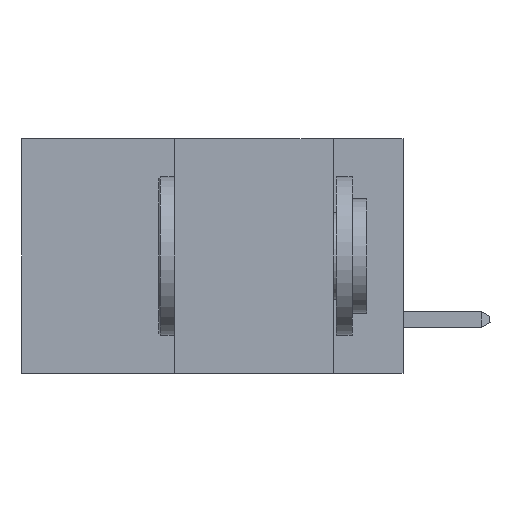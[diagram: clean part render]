
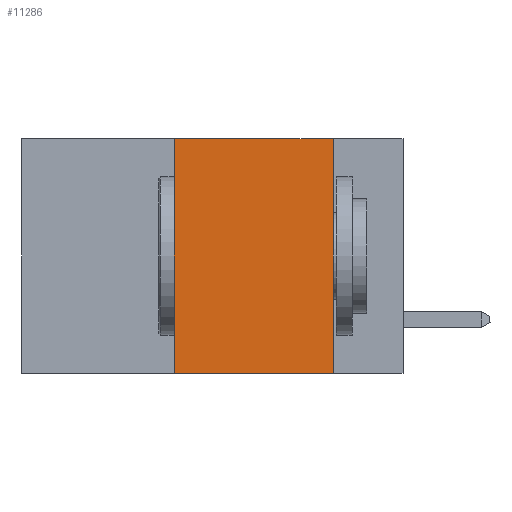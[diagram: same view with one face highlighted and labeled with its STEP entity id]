
A CAD part, left-side view. The second image highlights one B-rep face of the part: STEP entity #11286.
In plain terms, the highlighted planar face has unit normal (-1, 0, 0).
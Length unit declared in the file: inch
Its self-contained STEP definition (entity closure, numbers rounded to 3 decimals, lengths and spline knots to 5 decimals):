
#242 = DIRECTION ( 'NONE',  ( 0., -1., 0. ) ) ;
#502 = ORIENTED_EDGE ( 'NONE', *, *, #21085, .F. ) ;
#1889 = DIRECTION ( 'NONE',  ( 0., 0., 1. ) ) ;
#3334 = DIRECTION ( 'NONE',  ( 0., 0., -1. ) ) ;
#3608 = LINE ( 'NONE', #4258, #6875 ) ;
#3734 = ORIENTED_EDGE ( 'NONE', *, *, #17496, .F. ) ;
#4258 = CARTESIAN_POINT ( 'NONE',  ( 0., 0.6, 0. ) ) ;
#4529 = VECTOR ( 'NONE', #1889, 39.37008 ) ;
#4592 = CARTESIAN_POINT ( 'NONE',  ( 0., 0.11, 0. ) ) ;
#6875 = VECTOR ( 'NONE', #11330, 39.37008 ) ;
#7155 = VERTEX_POINT ( 'NONE', #19799 ) ;
#8104 = DIRECTION ( 'NONE',  ( 0., 0., -1. ) ) ;
#8480 = DIRECTION ( 'NONE',  ( 1., 0., 0. ) ) ;
#9555 = VECTOR ( 'NONE', #242, 39.37008 ) ;
#9782 = EDGE_CURVE ( 'NONE', #7155, #18331, #17671, .T. ) ;
#10585 = CARTESIAN_POINT ( 'NONE',  ( 0., 0.36, 0. ) ) ;
#11006 = CARTESIAN_POINT ( 'NONE',  ( 0., 0.11, 0. ) ) ;
#11286 = ADVANCED_FACE ( 'NONE', ( #14495 ), #16970, .F. ) ;
#11330 = DIRECTION ( 'NONE',  ( 0., -1., 0. ) ) ;
#11718 = CARTESIAN_POINT ( 'NONE',  ( 0., 0.6, -0.37 ) ) ;
#11725 = LINE ( 'NONE', #4592, #13318 ) ;
#11753 = ORIENTED_EDGE ( 'NONE', *, *, #9782, .T. ) ;
#12364 = VERTEX_POINT ( 'NONE', #11006 ) ;
#12646 = EDGE_CURVE ( 'NONE', #21403, #12364, #3608, .T. ) ;
#13174 = EDGE_LOOP ( 'NONE', ( #502, #13279, #3734, #11753 ) ) ;
#13279 = ORIENTED_EDGE ( 'NONE', *, *, #12646, .F. ) ;
#13318 = VECTOR ( 'NONE', #8104, 39.37008 ) ;
#14495 = FACE_OUTER_BOUND ( 'NONE', #13174, .T. ) ;
#15041 = CARTESIAN_POINT ( 'NONE',  ( 0., 0.6, 0. ) ) ;
#16970 = PLANE ( 'NONE',  #20222 ) ;
#17496 = EDGE_CURVE ( 'NONE', #7155, #21403, #18400, .T. ) ;
#17671 = LINE ( 'NONE', #11718, #9555 ) ;
#18160 = CARTESIAN_POINT ( 'NONE',  ( 0., 0.11, -0.37 ) ) ;
#18331 = VERTEX_POINT ( 'NONE', #18160 ) ;
#18400 = LINE ( 'NONE', #20968, #4529 ) ;
#19799 = CARTESIAN_POINT ( 'NONE',  ( 0., 0.36, -0.37 ) ) ;
#20222 = AXIS2_PLACEMENT_3D ( 'NONE', #15041, #8480, #3334 ) ;
#20968 = CARTESIAN_POINT ( 'NONE',  ( 0., 0.36, 0. ) ) ;
#21085 = EDGE_CURVE ( 'NONE', #12364, #18331, #11725, .T. ) ;
#21403 = VERTEX_POINT ( 'NONE', #10585 ) ;
